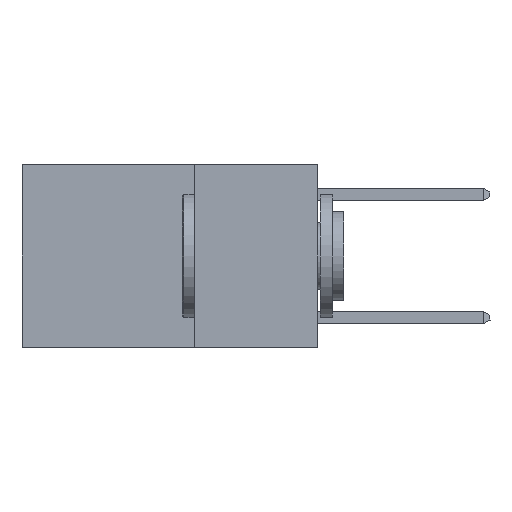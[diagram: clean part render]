
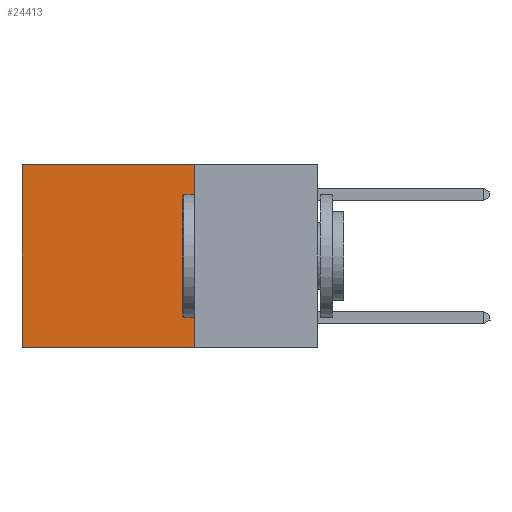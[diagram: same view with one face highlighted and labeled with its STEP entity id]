
A CAD part, left-side view. The second image highlights one B-rep face of the part: STEP entity #24413.
In plain terms, the highlighted planar face has unit normal (-1, 0, 0).
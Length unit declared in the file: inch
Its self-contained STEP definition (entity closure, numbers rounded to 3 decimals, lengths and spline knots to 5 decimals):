
#1895 = CARTESIAN_POINT ( 'NONE',  ( 0.2625, 0.25, 0. ) ) ;
#2193 = CARTESIAN_POINT ( 'NONE',  ( 0.2625, 0.6, 0. ) ) ;
#2444 = VECTOR ( 'NONE', #3861, 39.37008 ) ;
#3010 = EDGE_CURVE ( 'NONE', #13611, #12335, #11002, .T. ) ;
#3143 = AXIS2_PLACEMENT_3D ( 'NONE', #18009, #6771, #19905 ) ;
#3261 = ORIENTED_EDGE ( 'NONE', *, *, #12016, .T. ) ;
#3861 = DIRECTION ( 'NONE',  ( 0., 0., -1. ) ) ;
#3951 = VECTOR ( 'NONE', #12019, 39.37008 ) ;
#3963 = FACE_OUTER_BOUND ( 'NONE', #16823, .T. ) ;
#5323 = CARTESIAN_POINT ( 'NONE',  ( 0.2625, 0.25, -0.37 ) ) ;
#5815 = ORIENTED_EDGE ( 'NONE', *, *, #3010, .T. ) ;
#6462 = CARTESIAN_POINT ( 'NONE',  ( 0.2625, 0.6, 0. ) ) ;
#6771 = DIRECTION ( 'NONE',  ( 1., 0., 0. ) ) ;
#6858 = DIRECTION ( 'NONE',  ( 0., 1., 0. ) ) ;
#7199 = CARTESIAN_POINT ( 'NONE',  ( 0.2625, 0.6, -0.37 ) ) ;
#7542 = LINE ( 'NONE', #1895, #2444 ) ;
#8229 = VERTEX_POINT ( 'NONE', #22821 ) ;
#8418 = ORIENTED_EDGE ( 'NONE', *, *, #14528, .F. ) ;
#9268 = VECTOR ( 'NONE', #21483, 39.37008 ) ;
#11002 = LINE ( 'NONE', #6462, #9268 ) ;
#12016 = EDGE_CURVE ( 'NONE', #8229, #13611, #22820, .T. ) ;
#12019 = DIRECTION ( 'NONE',  ( 0., 1., 0. ) ) ;
#12335 = VERTEX_POINT ( 'NONE', #7199 ) ;
#12492 = EDGE_CURVE ( 'NONE', #8229, #13374, #7542, .T. ) ;
#12693 = ORIENTED_EDGE ( 'NONE', *, *, #12492, .F. ) ;
#13374 = VERTEX_POINT ( 'NONE', #5323 ) ;
#13611 = VERTEX_POINT ( 'NONE', #2193 ) ;
#13849 = VECTOR ( 'NONE', #6858, 39.37008 ) ;
#14528 = EDGE_CURVE ( 'NONE', #13374, #12335, #18889, .T. ) ;
#16196 = CARTESIAN_POINT ( 'NONE',  ( 0.2625, 0.25, -0.37 ) ) ;
#16823 = EDGE_LOOP ( 'NONE', ( #5815, #8418, #12693, #3261 ) ) ;
#18009 = CARTESIAN_POINT ( 'NONE',  ( 0.2625, 0.25, 0. ) ) ;
#18889 = LINE ( 'NONE', #16196, #13849 ) ;
#19535 = CARTESIAN_POINT ( 'NONE',  ( 0.2625, 0.25, 0. ) ) ;
#19819 = PLANE ( 'NONE',  #3143 ) ;
#19905 = DIRECTION ( 'NONE',  ( 0., 0., -1. ) ) ;
#21483 = DIRECTION ( 'NONE',  ( 0., 0., -1. ) ) ;
#22820 = LINE ( 'NONE', #19535, #3951 ) ;
#22821 = CARTESIAN_POINT ( 'NONE',  ( 0.2625, 0.25, 0. ) ) ;
#24413 = ADVANCED_FACE ( 'NONE', ( #3963 ), #19819, .F. ) ;
